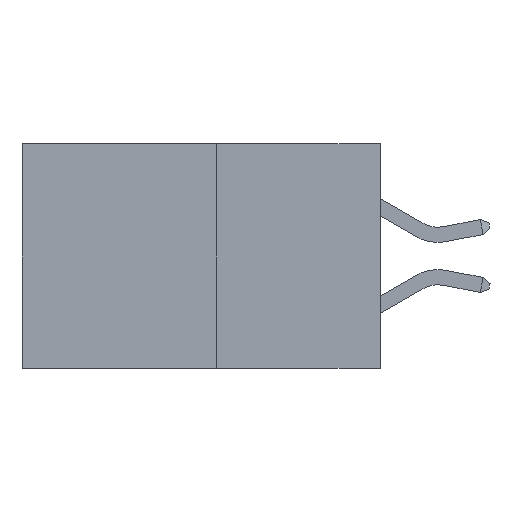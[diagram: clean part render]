
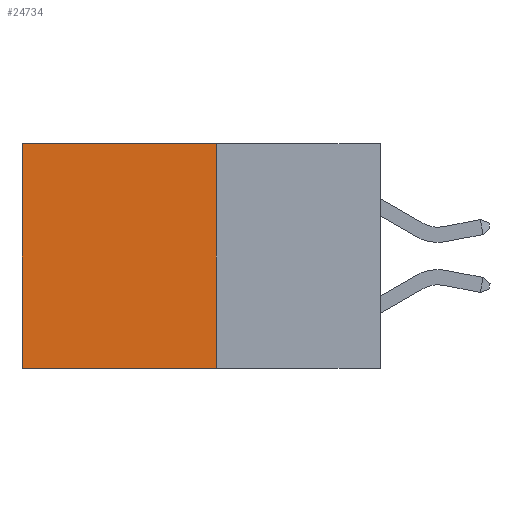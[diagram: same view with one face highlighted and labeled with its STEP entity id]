
A CAD part, left-side view. The second image highlights one B-rep face of the part: STEP entity #24734.
In plain terms, the highlighted planar face has unit normal (-1, 0, 0).
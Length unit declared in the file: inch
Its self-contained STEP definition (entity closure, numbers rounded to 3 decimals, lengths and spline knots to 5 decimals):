
#351 = VECTOR ( 'NONE', #15276, 39.37008 ) ;
#683 = CARTESIAN_POINT ( 'NONE',  ( 0.277, 0.27, 0. ) ) ;
#1747 = CARTESIAN_POINT ( 'NONE',  ( 0.277, 0.27, -0.37 ) ) ;
#2013 = CARTESIAN_POINT ( 'NONE',  ( 0.277, 0.27, -0.37 ) ) ;
#2756 = DIRECTION ( 'NONE',  ( 0., 1., 0. ) ) ;
#4024 = VECTOR ( 'NONE', #6815, 39.37008 ) ;
#4054 = DIRECTION ( 'NONE',  ( 1., 0., 0. ) ) ;
#5250 = ORIENTED_EDGE ( 'NONE', *, *, #24881, .T. ) ;
#6662 = CARTESIAN_POINT ( 'NONE',  ( 0.277, 0.59, -0.37 ) ) ;
#6815 = DIRECTION ( 'NONE',  ( 0., 1., 0. ) ) ;
#7134 = AXIS2_PLACEMENT_3D ( 'NONE', #1747, #4054, #19383 ) ;
#7280 = EDGE_CURVE ( 'NONE', #16655, #18237, #9909, .T. ) ;
#7408 = EDGE_LOOP ( 'NONE', ( #5250, #9654, #9245, #18072 ) ) ;
#8892 = DIRECTION ( 'NONE',  ( 0., 0., -1. ) ) ;
#9245 = ORIENTED_EDGE ( 'NONE', *, *, #28111, .F. ) ;
#9654 = ORIENTED_EDGE ( 'NONE', *, *, #11420, .F. ) ;
#9892 = VERTEX_POINT ( 'NONE', #17354 ) ;
#9909 = LINE ( 'NONE', #11136, #4024 ) ;
#10412 = VERTEX_POINT ( 'NONE', #27526 ) ;
#10659 = LINE ( 'NONE', #6662, #20888 ) ;
#11136 = CARTESIAN_POINT ( 'NONE',  ( 0.277, 0.27, 0. ) ) ;
#11420 = EDGE_CURVE ( 'NONE', #9892, #10412, #26647, .T. ) ;
#12728 = CARTESIAN_POINT ( 'NONE',  ( 0.277, 0.59, 0. ) ) ;
#15276 = DIRECTION ( 'NONE',  ( 0., 0., -1. ) ) ;
#16655 = VERTEX_POINT ( 'NONE', #683 ) ;
#17354 = CARTESIAN_POINT ( 'NONE',  ( 0.277, 0.27, -0.37 ) ) ;
#18072 = ORIENTED_EDGE ( 'NONE', *, *, #7280, .T. ) ;
#18153 = CARTESIAN_POINT ( 'NONE',  ( 0.277, 0.27, -0.37 ) ) ;
#18237 = VERTEX_POINT ( 'NONE', #12728 ) ;
#19383 = DIRECTION ( 'NONE',  ( 0., 0., -1. ) ) ;
#20888 = VECTOR ( 'NONE', #8892, 39.37008 ) ;
#20937 = VECTOR ( 'NONE', #2756, 39.37008 ) ;
#24734 = ADVANCED_FACE ( 'NONE', ( #24960 ), #27936, .F. ) ;
#24881 = EDGE_CURVE ( 'NONE', #18237, #10412, #10659, .T. ) ;
#24960 = FACE_OUTER_BOUND ( 'NONE', #7408, .T. ) ;
#26647 = LINE ( 'NONE', #18153, #20937 ) ;
#27526 = CARTESIAN_POINT ( 'NONE',  ( 0.277, 0.59, -0.37 ) ) ;
#27936 = PLANE ( 'NONE',  #7134 ) ;
#28060 = LINE ( 'NONE', #2013, #351 ) ;
#28111 = EDGE_CURVE ( 'NONE', #16655, #9892, #28060, .T. ) ;
